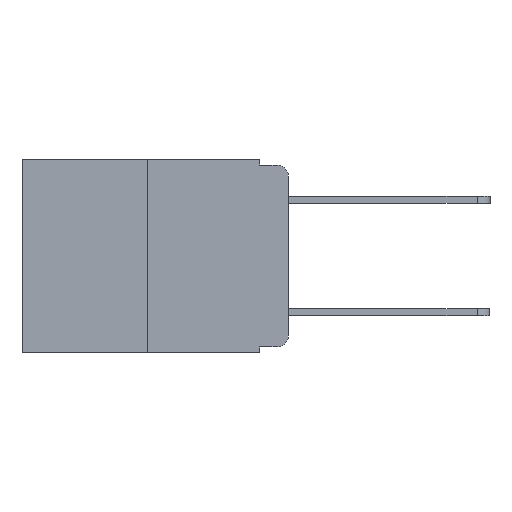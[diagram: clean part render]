
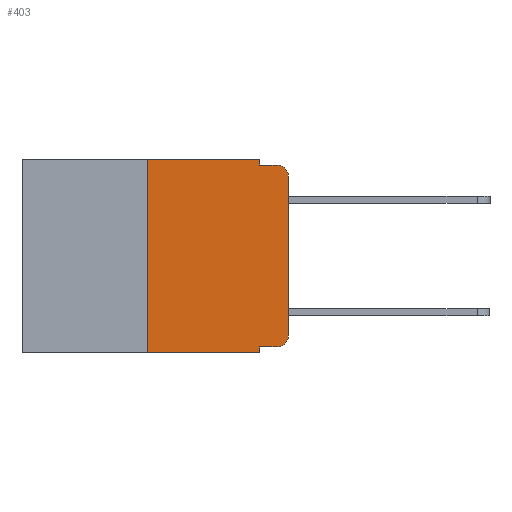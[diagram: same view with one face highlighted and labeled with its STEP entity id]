
A CAD part, left-side view. The second image highlights one B-rep face of the part: STEP entity #403.
In plain terms, the highlighted planar face has unit normal (-1, 0, 0).
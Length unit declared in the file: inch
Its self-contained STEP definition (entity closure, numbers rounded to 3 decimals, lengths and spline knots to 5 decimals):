
#84 = ORIENTED_EDGE ( 'NONE', *, *, #7704, .F. ) ;
#88 = DIRECTION ( 'NONE',  ( 0., 0., -1. ) ) ;
#170 = EDGE_CURVE ( 'NONE', #4234, #1712, #10230, .T. ) ;
#403 = ADVANCED_FACE ( 'NONE', ( #899 ), #8207, .F. ) ;
#899 = FACE_OUTER_BOUND ( 'NONE', #1416, .T. ) ;
#1011 = VECTOR ( 'NONE', #7729, 39.37008 ) ;
#1064 = CARTESIAN_POINT ( 'NONE',  ( 0., 0., -0.313 ) ) ;
#1091 = VERTEX_POINT ( 'NONE', #4423 ) ;
#1113 = VECTOR ( 'NONE', #4698, 39.37008 ) ;
#1388 = VERTEX_POINT ( 'NONE', #9225 ) ;
#1416 = EDGE_LOOP ( 'NONE', ( #6582, #9085, #8415, #84, #7766, #3577, #6472, #6987, #7524, #3587 ) ) ;
#1712 = VERTEX_POINT ( 'NONE', #4993 ) ;
#2008 = DIRECTION ( 'NONE',  ( 0., 0., 1. ) ) ;
#2040 = VECTOR ( 'NONE', #5581, 39.37008 ) ;
#2096 = VERTEX_POINT ( 'NONE', #6751 ) ;
#2097 = VERTEX_POINT ( 'NONE', #6894 ) ;
#2101 = CIRCLE ( 'NONE', #10128, 0.02 ) ;
#2172 = EDGE_CURVE ( 'NONE', #4234, #2097, #6501, .T. ) ;
#2200 = DIRECTION ( 'NONE',  ( -1., 0., 0. ) ) ;
#2539 = CARTESIAN_POINT ( 'NONE',  ( 0., 0.473, 0. ) ) ;
#2636 = VECTOR ( 'NONE', #3608, 39.37008 ) ;
#3015 = EDGE_CURVE ( 'NONE', #5911, #4054, #8849, .T. ) ;
#3221 = CARTESIAN_POINT ( 'NONE',  ( 0., 0.473, -0.343 ) ) ;
#3508 = LINE ( 'NONE', #11103, #1011 ) ;
#3577 = ORIENTED_EDGE ( 'NONE', *, *, #2172, .F. ) ;
#3587 = ORIENTED_EDGE ( 'NONE', *, *, #3015, .T. ) ;
#3608 = DIRECTION ( 'NONE',  ( 0., -1., 0. ) ) ;
#3622 = VECTOR ( 'NONE', #2008, 39.37008 ) ;
#3678 = DIRECTION ( 'NONE',  ( 0., -1., 0. ) ) ;
#3867 = AXIS2_PLACEMENT_3D ( 'NONE', #2539, #8076, #8777 ) ;
#4002 = DIRECTION ( 'NONE',  ( 0., 0., -1. ) ) ;
#4054 = VERTEX_POINT ( 'NONE', #1064 ) ;
#4234 = VERTEX_POINT ( 'NONE', #11264 ) ;
#4423 = CARTESIAN_POINT ( 'NONE',  ( 0., 0.051, 0. ) ) ;
#4626 = DIRECTION ( 'NONE',  ( 0., 0., -1. ) ) ;
#4677 = DIRECTION ( 'NONE',  ( -1., 0., 0. ) ) ;
#4686 = CARTESIAN_POINT ( 'NONE',  ( 0., 0.02, -0.313 ) ) ;
#4698 = DIRECTION ( 'NONE',  ( 0., -1., 0. ) ) ;
#4993 = CARTESIAN_POINT ( 'NONE',  ( 0., 0.051, -0.343 ) ) ;
#5003 = VECTOR ( 'NONE', #4002, 39.37008 ) ;
#5472 = EDGE_CURVE ( 'NONE', #6943, #2096, #2101, .T. ) ;
#5581 = DIRECTION ( 'NONE',  ( 0., -1., 0. ) ) ;
#5726 = CARTESIAN_POINT ( 'NONE',  ( 0., 0.25, 0. ) ) ;
#5802 = LINE ( 'NONE', #7183, #1113 ) ;
#5911 = VERTEX_POINT ( 'NONE', #9128 ) ;
#6016 = CARTESIAN_POINT ( 'NONE',  ( 0., 0.02, -0.03 ) ) ;
#6141 = DIRECTION ( 'NONE',  ( 0., 0., 1. ) ) ;
#6237 = CARTESIAN_POINT ( 'NONE',  ( 0., 0.051, -0.01 ) ) ;
#6460 = VERTEX_POINT ( 'NONE', #6237 ) ;
#6472 = ORIENTED_EDGE ( 'NONE', *, *, #170, .T. ) ;
#6501 = LINE ( 'NONE', #5726, #9004 ) ;
#6582 = ORIENTED_EDGE ( 'NONE', *, *, #9926, .T. ) ;
#6584 = EDGE_CURVE ( 'NONE', #6460, #2096, #5802, .T. ) ;
#6751 = CARTESIAN_POINT ( 'NONE',  ( 0., 0.02, -0.01 ) ) ;
#6894 = CARTESIAN_POINT ( 'NONE',  ( 0., 0.25, 0. ) ) ;
#6943 = VERTEX_POINT ( 'NONE', #10902 ) ;
#6987 = ORIENTED_EDGE ( 'NONE', *, *, #9406, .F. ) ;
#7097 = CARTESIAN_POINT ( 'NONE',  ( 0., 0., 0. ) ) ;
#7183 = CARTESIAN_POINT ( 'NONE',  ( 0., 0.051, -0.01 ) ) ;
#7235 = AXIS2_PLACEMENT_3D ( 'NONE', #4686, #4677, #4626 ) ;
#7524 = ORIENTED_EDGE ( 'NONE', *, *, #11109, .T. ) ;
#7704 = EDGE_CURVE ( 'NONE', #1091, #6460, #11199, .T. ) ;
#7729 = DIRECTION ( 'NONE',  ( 0., 0., -1. ) ) ;
#7766 = ORIENTED_EDGE ( 'NONE', *, *, #10872, .F. ) ;
#8076 = DIRECTION ( 'NONE',  ( 1., 0., 0. ) ) ;
#8207 = PLANE ( 'NONE',  #3867 ) ;
#8415 = ORIENTED_EDGE ( 'NONE', *, *, #6584, .F. ) ;
#8579 = LINE ( 'NONE', #8698, #8967 ) ;
#8623 = CARTESIAN_POINT ( 'NONE',  ( 0., 0.473, 0. ) ) ;
#8698 = CARTESIAN_POINT ( 'NONE',  ( 0., 0.051, -0.333 ) ) ;
#8777 = DIRECTION ( 'NONE',  ( 0., 0., -1. ) ) ;
#8849 = CIRCLE ( 'NONE', #7235, 0.02 ) ;
#8967 = VECTOR ( 'NONE', #3678, 39.37008 ) ;
#9004 = VECTOR ( 'NONE', #6141, 39.37008 ) ;
#9032 = CARTESIAN_POINT ( 'NONE',  ( 0., 0.051, 0. ) ) ;
#9085 = ORIENTED_EDGE ( 'NONE', *, *, #5472, .T. ) ;
#9109 = LINE ( 'NONE', #8623, #2636 ) ;
#9128 = CARTESIAN_POINT ( 'NONE',  ( 0., 0.02, -0.333 ) ) ;
#9225 = CARTESIAN_POINT ( 'NONE',  ( 0., 0.051, -0.333 ) ) ;
#9406 = EDGE_CURVE ( 'NONE', #1388, #1712, #3508, .T. ) ;
#9926 = EDGE_CURVE ( 'NONE', #4054, #6943, #10038, .T. ) ;
#10038 = LINE ( 'NONE', #7097, #3622 ) ;
#10128 = AXIS2_PLACEMENT_3D ( 'NONE', #6016, #2200, #88 ) ;
#10230 = LINE ( 'NONE', #3221, #2040 ) ;
#10872 = EDGE_CURVE ( 'NONE', #2097, #1091, #9109, .T. ) ;
#10902 = CARTESIAN_POINT ( 'NONE',  ( 0., 0., -0.03 ) ) ;
#11103 = CARTESIAN_POINT ( 'NONE',  ( 0., 0.051, 0. ) ) ;
#11109 = EDGE_CURVE ( 'NONE', #1388, #5911, #8579, .T. ) ;
#11199 = LINE ( 'NONE', #9032, #5003 ) ;
#11264 = CARTESIAN_POINT ( 'NONE',  ( 0., 0.25, -0.343 ) ) ;
